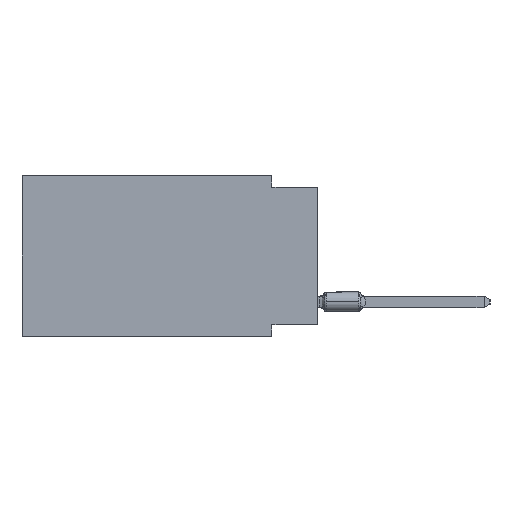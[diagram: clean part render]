
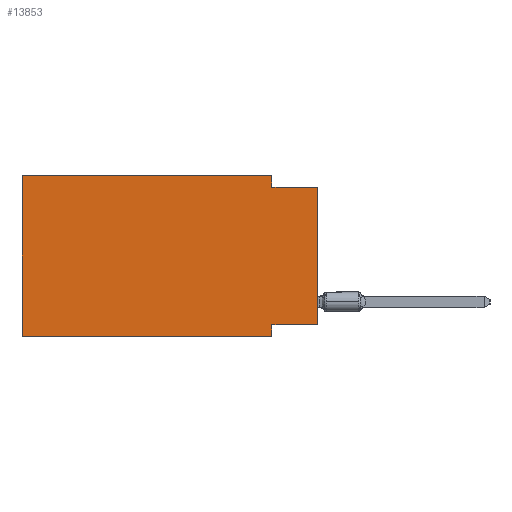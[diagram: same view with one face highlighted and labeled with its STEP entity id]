
A CAD part, left-side view. The second image highlights one B-rep face of the part: STEP entity #13853.
In plain terms, the highlighted planar face has unit normal (-1, 0, 0).
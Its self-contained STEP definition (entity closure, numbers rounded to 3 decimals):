
#165 = CARTESIAN_POINT ( 'NONE',  ( 0., 0., -8.255 ) ) ;
#608 = ORIENTED_EDGE ( 'NONE', *, *, #11941, .F. ) ;
#1564 = CARTESIAN_POINT ( 'NONE',  ( 0., 0., -0.635 ) ) ;
#2432 = CARTESIAN_POINT ( 'NONE',  ( 0., 0., 0. ) ) ;
#3468 = ORIENTED_EDGE ( 'NONE', *, *, #8998, .F. ) ;
#3497 = EDGE_CURVE ( 'NONE', #11002, #26225, #19851, .T. ) ;
#3604 = PLANE ( 'NONE',  #7973 ) ;
#3748 = CARTESIAN_POINT ( 'NONE',  ( 0., 16.383, 0. ) ) ;
#3992 = CARTESIAN_POINT ( 'NONE',  ( 0., 2.54, -8.255 ) ) ;
#4440 = DIRECTION ( 'NONE',  ( 0., 1., 0. ) ) ;
#4507 = DIRECTION ( 'NONE',  ( 0., 0., -1. ) ) ;
#5402 = EDGE_CURVE ( 'NONE', #24436, #20348, #5532, .T. ) ;
#5447 = ORIENTED_EDGE ( 'NONE', *, *, #11530, .T. ) ;
#5472 = LINE ( 'NONE', #14400, #20135 ) ;
#5532 = LINE ( 'NONE', #27767, #6213 ) ;
#5622 = LINE ( 'NONE', #8398, #13166 ) ;
#6213 = VECTOR ( 'NONE', #7724, 1000. ) ;
#6847 = LINE ( 'NONE', #8907, #10929 ) ;
#7724 = DIRECTION ( 'NONE',  ( 0., -1., 0. ) ) ;
#7973 = AXIS2_PLACEMENT_3D ( 'NONE', #3748, #10170, #8430 ) ;
#8398 = CARTESIAN_POINT ( 'NONE',  ( 0., 16.383, -8.89 ) ) ;
#8430 = DIRECTION ( 'NONE',  ( 0., 0., -1. ) ) ;
#8845 = LINE ( 'NONE', #24922, #14889 ) ;
#8878 = LINE ( 'NONE', #2432, #14476 ) ;
#8907 = CARTESIAN_POINT ( 'NONE',  ( 0., 2.54, -8.89 ) ) ;
#8998 = EDGE_CURVE ( 'NONE', #21186, #24436, #15418, .T. ) ;
#9314 = ORIENTED_EDGE ( 'NONE', *, *, #5402, .F. ) ;
#10170 = DIRECTION ( 'NONE',  ( 1., 0., 0. ) ) ;
#10929 = VECTOR ( 'NONE', #4507, 1000. ) ;
#11002 = VERTEX_POINT ( 'NONE', #17542 ) ;
#11530 = EDGE_CURVE ( 'NONE', #27667, #26225, #8878, .T. ) ;
#11941 = EDGE_CURVE ( 'NONE', #27667, #18176, #8845, .T. ) ;
#12374 = FACE_OUTER_BOUND ( 'NONE', #17598, .T. ) ;
#13166 = VECTOR ( 'NONE', #28000, 1000. ) ;
#13374 = ORIENTED_EDGE ( 'NONE', *, *, #3497, .F. ) ;
#13396 = DIRECTION ( 'NONE',  ( 0., 0., 1. ) ) ;
#13853 = ADVANCED_FACE ( 'NONE', ( #12374 ), #3604, .F. ) ;
#14315 = EDGE_CURVE ( 'NONE', #20348, #11002, #5472, .T. ) ;
#14400 = CARTESIAN_POINT ( 'NONE',  ( 0., 2.54, 0. ) ) ;
#14476 = VECTOR ( 'NONE', #13396, 1000. ) ;
#14889 = VECTOR ( 'NONE', #4440, 1000. ) ;
#15418 = LINE ( 'NONE', #24476, #20860 ) ;
#15507 = EDGE_CURVE ( 'NONE', #21186, #28258, #5622, .T. ) ;
#15705 = DIRECTION ( 'NONE',  ( 0., 0., 1. ) ) ;
#15878 = VECTOR ( 'NONE', #25998, 1000. ) ;
#16137 = CARTESIAN_POINT ( 'NONE',  ( 0., 16.383, 0. ) ) ;
#17542 = CARTESIAN_POINT ( 'NONE',  ( 0., 2.54, -0.635 ) ) ;
#17598 = EDGE_LOOP ( 'NONE', ( #5447, #13374, #18464, #9314, #3468, #23126, #25705, #608 ) ) ;
#18176 = VERTEX_POINT ( 'NONE', #3992 ) ;
#18464 = ORIENTED_EDGE ( 'NONE', *, *, #14315, .F. ) ;
#19739 = CARTESIAN_POINT ( 'NONE',  ( 0., 0., -0.635 ) ) ;
#19851 = LINE ( 'NONE', #1564, #15878 ) ;
#19958 = CARTESIAN_POINT ( 'NONE',  ( 0., 2.54, -8.89 ) ) ;
#20135 = VECTOR ( 'NONE', #23331, 1000. ) ;
#20348 = VERTEX_POINT ( 'NONE', #21082 ) ;
#20860 = VECTOR ( 'NONE', #15705, 1000. ) ;
#21082 = CARTESIAN_POINT ( 'NONE',  ( 0., 2.54, 0. ) ) ;
#21186 = VERTEX_POINT ( 'NONE', #25637 ) ;
#21933 = EDGE_CURVE ( 'NONE', #18176, #28258, #6847, .T. ) ;
#23126 = ORIENTED_EDGE ( 'NONE', *, *, #15507, .T. ) ;
#23331 = DIRECTION ( 'NONE',  ( 0., 0., -1. ) ) ;
#24436 = VERTEX_POINT ( 'NONE', #16137 ) ;
#24476 = CARTESIAN_POINT ( 'NONE',  ( 0., 16.383, 0. ) ) ;
#24922 = CARTESIAN_POINT ( 'NONE',  ( 0., 0., -8.255 ) ) ;
#25637 = CARTESIAN_POINT ( 'NONE',  ( 0., 16.383, -8.89 ) ) ;
#25705 = ORIENTED_EDGE ( 'NONE', *, *, #21933, .F. ) ;
#25998 = DIRECTION ( 'NONE',  ( 0., -1., 0. ) ) ;
#26225 = VERTEX_POINT ( 'NONE', #19739 ) ;
#27667 = VERTEX_POINT ( 'NONE', #165 ) ;
#27767 = CARTESIAN_POINT ( 'NONE',  ( 0., 16.383, 0. ) ) ;
#28000 = DIRECTION ( 'NONE',  ( 0., -1., 0. ) ) ;
#28258 = VERTEX_POINT ( 'NONE', #19958 ) ;
